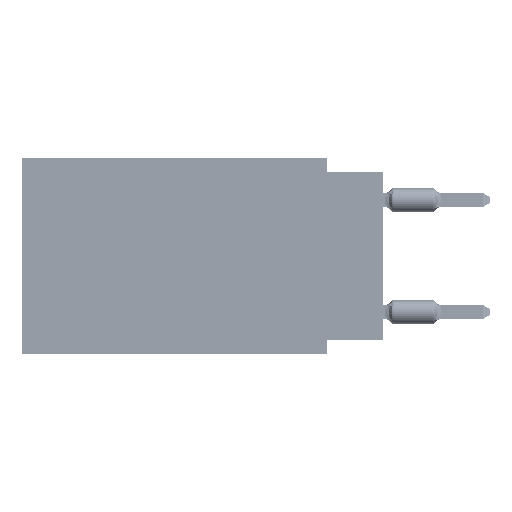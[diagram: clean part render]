
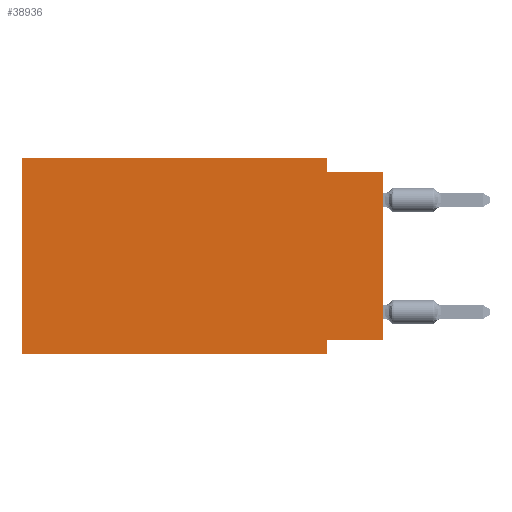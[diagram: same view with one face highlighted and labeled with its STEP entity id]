
A CAD part, left-side view. The second image highlights one B-rep face of the part: STEP entity #38936.
In plain terms, the highlighted planar face has unit normal (-1, 0, 0).
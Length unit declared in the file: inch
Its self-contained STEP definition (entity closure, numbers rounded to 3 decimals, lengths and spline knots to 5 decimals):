
#2107 = CARTESIAN_POINT ( 'NONE',  ( 0., 0.645, -0.35 ) ) ;
#3673 = CARTESIAN_POINT ( 'NONE',  ( 0., 0.1, -0.35 ) ) ;
#3816 = ORIENTED_EDGE ( 'NONE', *, *, #20980, .T. ) ;
#4230 = DIRECTION ( 'NONE',  ( 0., 0., -1. ) ) ;
#5596 = FACE_OUTER_BOUND ( 'NONE', #50584, .T. ) ;
#10678 = DIRECTION ( 'NONE',  ( 0., 0., 1. ) ) ;
#12753 = CARTESIAN_POINT ( 'NONE',  ( 0., 0.1, 0. ) ) ;
#14029 = EDGE_CURVE ( 'NONE', #46460, #79740, #75591, .T. ) ;
#16580 = CARTESIAN_POINT ( 'NONE',  ( 0., 0.645, 0. ) ) ;
#18110 = VECTOR ( 'NONE', #4230, 39.37008 ) ;
#18736 = DIRECTION ( 'NONE',  ( 0., -1., 0. ) ) ;
#19577 = CARTESIAN_POINT ( 'NONE',  ( 0., 0., 0. ) ) ;
#20980 = EDGE_CURVE ( 'NONE', #34973, #51192, #92176, .T. ) ;
#22683 = CARTESIAN_POINT ( 'NONE',  ( 0., 0., -0.325 ) ) ;
#27955 = EDGE_CURVE ( 'NONE', #61275, #111373, #48292, .T. ) ;
#30889 = DIRECTION ( 'NONE',  ( 0., -1., 0. ) ) ;
#34505 = EDGE_CURVE ( 'NONE', #76334, #61275, #67063, .T. ) ;
#34973 = VERTEX_POINT ( 'NONE', #95750 ) ;
#36921 = VECTOR ( 'NONE', #10678, 39.37008 ) ;
#38256 = CARTESIAN_POINT ( 'NONE',  ( 0., 0., -0.025 ) ) ;
#38936 = ADVANCED_FACE ( 'NONE', ( #5596 ), #94511, .F. ) ;
#40937 = LINE ( 'NONE', #95428, #72454 ) ;
#41763 = EDGE_CURVE ( 'NONE', #79740, #51192, #58186, .T. ) ;
#42678 = LINE ( 'NONE', #16580, #47442 ) ;
#46460 = VERTEX_POINT ( 'NONE', #22683 ) ;
#47442 = VECTOR ( 'NONE', #69348, 39.37008 ) ;
#48292 = LINE ( 'NONE', #38256, #93737 ) ;
#49446 = EDGE_CURVE ( 'NONE', #64341, #76334, #40937, .T. ) ;
#50584 = EDGE_LOOP ( 'NONE', ( #66849, #68031, #102156, #99629, #116531, #3816, #102190, #72759 ) ) ;
#51192 = VERTEX_POINT ( 'NONE', #58256 ) ;
#58186 = LINE ( 'NONE', #3673, #62227 ) ;
#58256 = CARTESIAN_POINT ( 'NONE',  ( 0., 0.1, -0.35 ) ) ;
#60121 = DIRECTION ( 'NONE',  ( 1., 0., 0. ) ) ;
#60561 = VECTOR ( 'NONE', #66120, 39.37008 ) ;
#61275 = VERTEX_POINT ( 'NONE', #115906 ) ;
#62227 = VECTOR ( 'NONE', #102623, 39.37008 ) ;
#64341 = VERTEX_POINT ( 'NONE', #86667 ) ;
#65605 = AXIS2_PLACEMENT_3D ( 'NONE', #84435, #60121, #114003 ) ;
#65893 = CARTESIAN_POINT ( 'NONE',  ( 0., 0.1, 0. ) ) ;
#66120 = DIRECTION ( 'NONE',  ( 0., 1., 0. ) ) ;
#66849 = ORIENTED_EDGE ( 'NONE', *, *, #109569, .T. ) ;
#67063 = LINE ( 'NONE', #65893, #18110 ) ;
#67410 = CARTESIAN_POINT ( 'NONE',  ( 0., 0., -0.025 ) ) ;
#68031 = ORIENTED_EDGE ( 'NONE', *, *, #27955, .F. ) ;
#69348 = DIRECTION ( 'NONE',  ( 0., 0., 1. ) ) ;
#72454 = VECTOR ( 'NONE', #30889, 39.37008 ) ;
#72759 = ORIENTED_EDGE ( 'NONE', *, *, #14029, .F. ) ;
#74384 = DIRECTION ( 'NONE',  ( 0., -1., 0. ) ) ;
#75591 = LINE ( 'NONE', #111723, #60561 ) ;
#76334 = VERTEX_POINT ( 'NONE', #12753 ) ;
#79740 = VERTEX_POINT ( 'NONE', #100405 ) ;
#80772 = VECTOR ( 'NONE', #18736, 39.37008 ) ;
#84435 = CARTESIAN_POINT ( 'NONE',  ( 0., 0.645, 0. ) ) ;
#86667 = CARTESIAN_POINT ( 'NONE',  ( 0., 0.645, 0. ) ) ;
#86816 = EDGE_CURVE ( 'NONE', #34973, #64341, #42678, .T. ) ;
#92176 = LINE ( 'NONE', #2107, #80772 ) ;
#92462 = LINE ( 'NONE', #19577, #36921 ) ;
#93737 = VECTOR ( 'NONE', #74384, 39.37008 ) ;
#94511 = PLANE ( 'NONE',  #65605 ) ;
#95428 = CARTESIAN_POINT ( 'NONE',  ( 0., 0.645, 0. ) ) ;
#95750 = CARTESIAN_POINT ( 'NONE',  ( 0., 0.645, -0.35 ) ) ;
#99629 = ORIENTED_EDGE ( 'NONE', *, *, #49446, .F. ) ;
#100405 = CARTESIAN_POINT ( 'NONE',  ( 0., 0.1, -0.325 ) ) ;
#102156 = ORIENTED_EDGE ( 'NONE', *, *, #34505, .F. ) ;
#102190 = ORIENTED_EDGE ( 'NONE', *, *, #41763, .F. ) ;
#102623 = DIRECTION ( 'NONE',  ( 0., 0., -1. ) ) ;
#109569 = EDGE_CURVE ( 'NONE', #46460, #111373, #92462, .T. ) ;
#111373 = VERTEX_POINT ( 'NONE', #67410 ) ;
#111723 = CARTESIAN_POINT ( 'NONE',  ( 0., 0., -0.325 ) ) ;
#114003 = DIRECTION ( 'NONE',  ( 0., 0., -1. ) ) ;
#115906 = CARTESIAN_POINT ( 'NONE',  ( 0., 0.1, -0.025 ) ) ;
#116531 = ORIENTED_EDGE ( 'NONE', *, *, #86816, .F. ) ;
